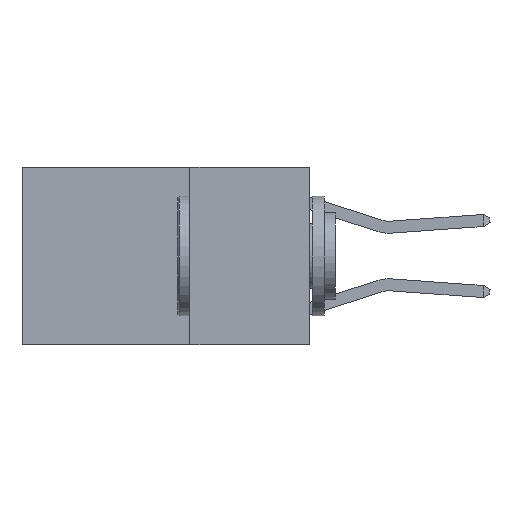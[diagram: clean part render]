
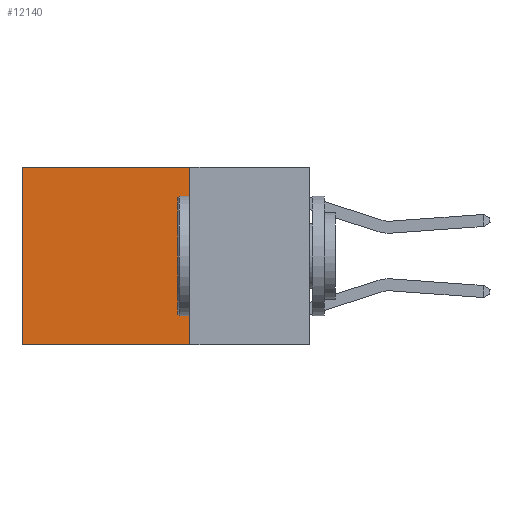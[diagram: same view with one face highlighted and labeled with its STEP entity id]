
A CAD part, left-side view. The second image highlights one B-rep face of the part: STEP entity #12140.
In plain terms, the highlighted planar face has unit normal (-1, 0, 0).
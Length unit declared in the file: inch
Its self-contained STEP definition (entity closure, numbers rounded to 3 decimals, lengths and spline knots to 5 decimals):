
#220 = DIRECTION ( 'NONE',  ( 1., 0., 0. ) ) ;
#350 = PLANE ( 'NONE',  #3653 ) ;
#629 = ORIENTED_EDGE ( 'NONE', *, *, #936, .T. ) ;
#862 = VERTEX_POINT ( 'NONE', #2356 ) ;
#936 = EDGE_CURVE ( 'NONE', #6580, #12982, #13542, .T. ) ;
#1542 = DIRECTION ( 'NONE',  ( 0., 0., -1. ) ) ;
#2356 = CARTESIAN_POINT ( 'NONE',  ( 0.2625, 0.25, -0.37 ) ) ;
#2498 = LINE ( 'NONE', #3811, #2898 ) ;
#2898 = VECTOR ( 'NONE', #1542, 39.37008 ) ;
#3143 = EDGE_CURVE ( 'NONE', #862, #5121, #4688, .T. ) ;
#3388 = CARTESIAN_POINT ( 'NONE',  ( 0.2625, 0.25, 0. ) ) ;
#3535 = FACE_OUTER_BOUND ( 'NONE', #4979, .T. ) ;
#3653 = AXIS2_PLACEMENT_3D ( 'NONE', #5685, #220, #3750 ) ;
#3750 = DIRECTION ( 'NONE',  ( 0., 0., -1. ) ) ;
#3811 = CARTESIAN_POINT ( 'NONE',  ( 0.2625, 0.25, 0. ) ) ;
#4116 = CARTESIAN_POINT ( 'NONE',  ( 0.2625, 0.6, -0.37 ) ) ;
#4688 = LINE ( 'NONE', #8179, #12885 ) ;
#4979 = EDGE_LOOP ( 'NONE', ( #6781, #13730, #9203, #629 ) ) ;
#5121 = VERTEX_POINT ( 'NONE', #4116 ) ;
#5685 = CARTESIAN_POINT ( 'NONE',  ( 0.2625, 0.25, 0. ) ) ;
#5724 = EDGE_CURVE ( 'NONE', #12982, #5121, #12417, .T. ) ;
#6580 = VERTEX_POINT ( 'NONE', #10222 ) ;
#6781 = ORIENTED_EDGE ( 'NONE', *, *, #5724, .T. ) ;
#7915 = DIRECTION ( 'NONE',  ( 0., 1., 0. ) ) ;
#8179 = CARTESIAN_POINT ( 'NONE',  ( 0.2625, 0.25, -0.37 ) ) ;
#8504 = EDGE_CURVE ( 'NONE', #6580, #862, #2498, .T. ) ;
#9132 = CARTESIAN_POINT ( 'NONE',  ( 0.2625, 0.6, 0. ) ) ;
#9203 = ORIENTED_EDGE ( 'NONE', *, *, #8504, .F. ) ;
#9288 = DIRECTION ( 'NONE',  ( 0., 1., 0. ) ) ;
#10204 = DIRECTION ( 'NONE',  ( 0., 0., -1. ) ) ;
#10222 = CARTESIAN_POINT ( 'NONE',  ( 0.2625, 0.25, 0. ) ) ;
#12140 = ADVANCED_FACE ( 'NONE', ( #3535 ), #350, .F. ) ;
#12284 = CARTESIAN_POINT ( 'NONE',  ( 0.2625, 0.6, 0. ) ) ;
#12296 = VECTOR ( 'NONE', #10204, 39.37008 ) ;
#12417 = LINE ( 'NONE', #12284, #12296 ) ;
#12885 = VECTOR ( 'NONE', #9288, 39.37008 ) ;
#12982 = VERTEX_POINT ( 'NONE', #9132 ) ;
#13219 = VECTOR ( 'NONE', #7915, 39.37008 ) ;
#13542 = LINE ( 'NONE', #3388, #13219 ) ;
#13730 = ORIENTED_EDGE ( 'NONE', *, *, #3143, .F. ) ;
